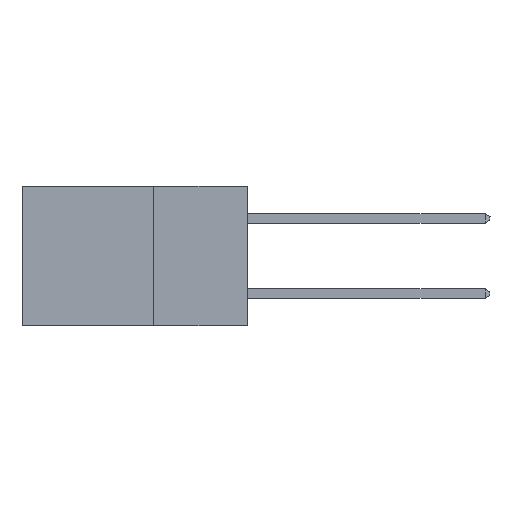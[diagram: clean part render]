
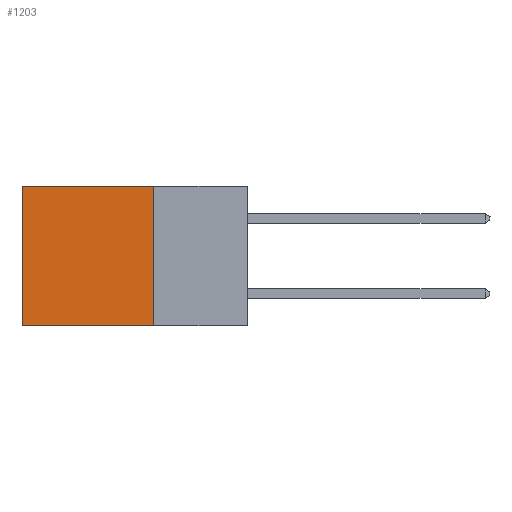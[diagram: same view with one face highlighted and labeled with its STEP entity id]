
A CAD part, left-side view. The second image highlights one B-rep face of the part: STEP entity #1203.
In plain terms, the highlighted planar face has unit normal (-1, 0, 0).
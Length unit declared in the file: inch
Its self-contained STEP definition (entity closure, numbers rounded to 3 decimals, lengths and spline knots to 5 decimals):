
#1203 = ADVANCED_FACE ( 'NONE', ( #12974 ), #12586, .F. ) ;
#2254 = CARTESIAN_POINT ( 'NONE',  ( 0.2615, 0.6, -0.37 ) ) ;
#3051 = CARTESIAN_POINT ( 'NONE',  ( 0.2615, 0.25, -0.37 ) ) ;
#3074 = VECTOR ( 'NONE', #21542, 39.37008 ) ;
#3492 = VECTOR ( 'NONE', #15026, 39.37008 ) ;
#4698 = EDGE_CURVE ( 'NONE', #21424, #24450, #22706, .T. ) ;
#4999 = DIRECTION ( 'NONE',  ( 0., 0., -1. ) ) ;
#6005 = AXIS2_PLACEMENT_3D ( 'NONE', #19073, #14648, #18678 ) ;
#6248 = VERTEX_POINT ( 'NONE', #7468 ) ;
#6440 = CARTESIAN_POINT ( 'NONE',  ( 0.2615, 0.6, 0. ) ) ;
#7468 = CARTESIAN_POINT ( 'NONE',  ( 0.2615, 0.6, -0.37 ) ) ;
#7949 = VECTOR ( 'NONE', #4999, 39.37008 ) ;
#8812 = CARTESIAN_POINT ( 'NONE',  ( 0.2615, 0.25, -0.37 ) ) ;
#9400 = ORIENTED_EDGE ( 'NONE', *, *, #18884, .T. ) ;
#9405 = ORIENTED_EDGE ( 'NONE', *, *, #23425, .F. ) ;
#9475 = ORIENTED_EDGE ( 'NONE', *, *, #4698, .F. ) ;
#9616 = CARTESIAN_POINT ( 'NONE',  ( 0.2615, 0.25, -0.37 ) ) ;
#9897 = CARTESIAN_POINT ( 'NONE',  ( 0.2615, 0.25, 0. ) ) ;
#11464 = LINE ( 'NONE', #9897, #3074 ) ;
#11720 = LINE ( 'NONE', #2254, #14505 ) ;
#12586 = PLANE ( 'NONE',  #6005 ) ;
#12974 = FACE_OUTER_BOUND ( 'NONE', #18307, .T. ) ;
#14505 = VECTOR ( 'NONE', #23840, 39.37008 ) ;
#14648 = DIRECTION ( 'NONE',  ( 1., 0., 0. ) ) ;
#14855 = EDGE_CURVE ( 'NONE', #21424, #25111, #11464, .T. ) ;
#15026 = DIRECTION ( 'NONE',  ( 0., 1., 0. ) ) ;
#17594 = CARTESIAN_POINT ( 'NONE',  ( 0.2615, 0.25, 0. ) ) ;
#18307 = EDGE_LOOP ( 'NONE', ( #9400, #9405, #9475, #23192 ) ) ;
#18678 = DIRECTION ( 'NONE',  ( 0., 0., -1. ) ) ;
#18884 = EDGE_CURVE ( 'NONE', #25111, #6248, #11720, .T. ) ;
#19073 = CARTESIAN_POINT ( 'NONE',  ( 0.2615, 0.25, -0.37 ) ) ;
#21424 = VERTEX_POINT ( 'NONE', #17594 ) ;
#21542 = DIRECTION ( 'NONE',  ( 0., 1., 0. ) ) ;
#22706 = LINE ( 'NONE', #3051, #7949 ) ;
#23192 = ORIENTED_EDGE ( 'NONE', *, *, #14855, .T. ) ;
#23425 = EDGE_CURVE ( 'NONE', #24450, #6248, #24835, .T. ) ;
#23840 = DIRECTION ( 'NONE',  ( 0., 0., -1. ) ) ;
#24450 = VERTEX_POINT ( 'NONE', #9616 ) ;
#24835 = LINE ( 'NONE', #8812, #3492 ) ;
#25111 = VERTEX_POINT ( 'NONE', #6440 ) ;
